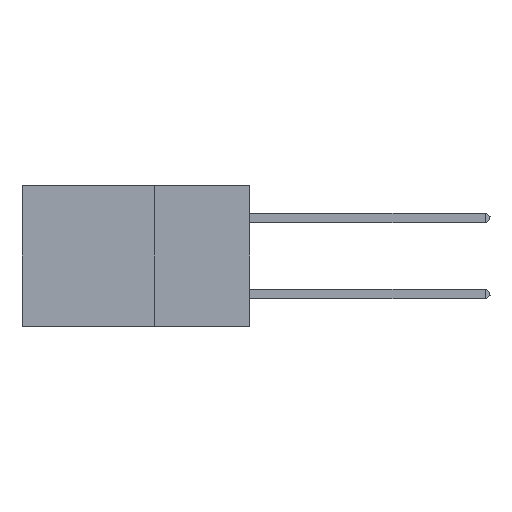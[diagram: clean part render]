
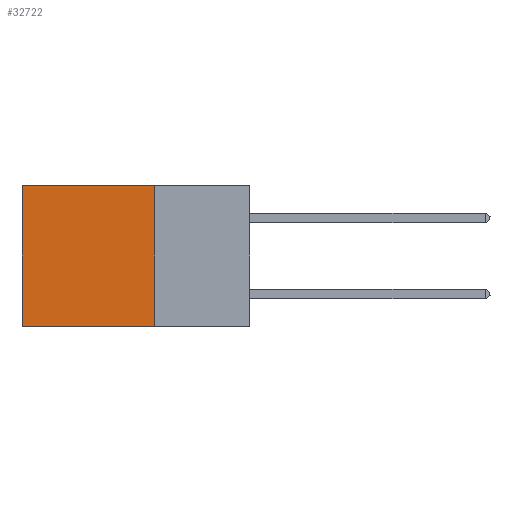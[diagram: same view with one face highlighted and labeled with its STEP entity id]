
A CAD part, left-side view. The second image highlights one B-rep face of the part: STEP entity #32722.
In plain terms, the highlighted planar face has unit normal (-1, 0, 0).
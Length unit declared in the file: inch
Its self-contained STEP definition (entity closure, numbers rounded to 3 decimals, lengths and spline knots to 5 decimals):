
#111 = LINE ( 'NONE', #25229, #27615 ) ;
#751 = VECTOR ( 'NONE', #21104, 39.37008 ) ;
#2361 = VERTEX_POINT ( 'NONE', #18587 ) ;
#2770 = DIRECTION ( 'NONE',  ( 0., 1., 0. ) ) ;
#3544 = FACE_OUTER_BOUND ( 'NONE', #27160, .T. ) ;
#5372 = VERTEX_POINT ( 'NONE', #31894 ) ;
#7346 = LINE ( 'NONE', #19290, #29225 ) ;
#7552 = AXIS2_PLACEMENT_3D ( 'NONE', #28608, #12138, #31343 ) ;
#8929 = LINE ( 'NONE', #26600, #751 ) ;
#9411 = PLANE ( 'NONE',  #7552 ) ;
#10067 = EDGE_CURVE ( 'NONE', #14162, #2361, #8929, .T. ) ;
#11466 = ORIENTED_EDGE ( 'NONE', *, *, #23828, .T. ) ;
#11507 = DIRECTION ( 'NONE',  ( 0., 0., -1. ) ) ;
#11811 = CARTESIAN_POINT ( 'NONE',  ( 0.2875, 0.25, 0. ) ) ;
#12138 = DIRECTION ( 'NONE',  ( 1., 0., 0. ) ) ;
#14162 = VERTEX_POINT ( 'NONE', #17924 ) ;
#15929 = DIRECTION ( 'NONE',  ( 0., 0., -1. ) ) ;
#17924 = CARTESIAN_POINT ( 'NONE',  ( 0.2875, 0.25, -0.37 ) ) ;
#18587 = CARTESIAN_POINT ( 'NONE',  ( 0.2875, 0.6, -0.37 ) ) ;
#19290 = CARTESIAN_POINT ( 'NONE',  ( 0.2875, 0.25, 0. ) ) ;
#21104 = DIRECTION ( 'NONE',  ( 0., 1., 0. ) ) ;
#22128 = LINE ( 'NONE', #32338, #29401 ) ;
#23124 = ORIENTED_EDGE ( 'NONE', *, *, #24809, .F. ) ;
#23828 = EDGE_CURVE ( 'NONE', #5372, #2361, #22128, .T. ) ;
#24809 = EDGE_CURVE ( 'NONE', #25550, #14162, #111, .T. ) ;
#24857 = ORIENTED_EDGE ( 'NONE', *, *, #33615, .T. ) ;
#25229 = CARTESIAN_POINT ( 'NONE',  ( 0.2875, 0.25, 0. ) ) ;
#25550 = VERTEX_POINT ( 'NONE', #11811 ) ;
#26600 = CARTESIAN_POINT ( 'NONE',  ( 0.2875, 0.25, -0.37 ) ) ;
#27160 = EDGE_LOOP ( 'NONE', ( #11466, #33105, #23124, #24857 ) ) ;
#27615 = VECTOR ( 'NONE', #11507, 39.37008 ) ;
#28608 = CARTESIAN_POINT ( 'NONE',  ( 0.2875, 0.25, 0. ) ) ;
#29225 = VECTOR ( 'NONE', #2770, 39.37008 ) ;
#29401 = VECTOR ( 'NONE', #15929, 39.37008 ) ;
#31343 = DIRECTION ( 'NONE',  ( 0., 0., -1. ) ) ;
#31894 = CARTESIAN_POINT ( 'NONE',  ( 0.2875, 0.6, 0. ) ) ;
#32338 = CARTESIAN_POINT ( 'NONE',  ( 0.2875, 0.6, 0. ) ) ;
#32722 = ADVANCED_FACE ( 'NONE', ( #3544 ), #9411, .F. ) ;
#33105 = ORIENTED_EDGE ( 'NONE', *, *, #10067, .F. ) ;
#33615 = EDGE_CURVE ( 'NONE', #25550, #5372, #7346, .T. ) ;
